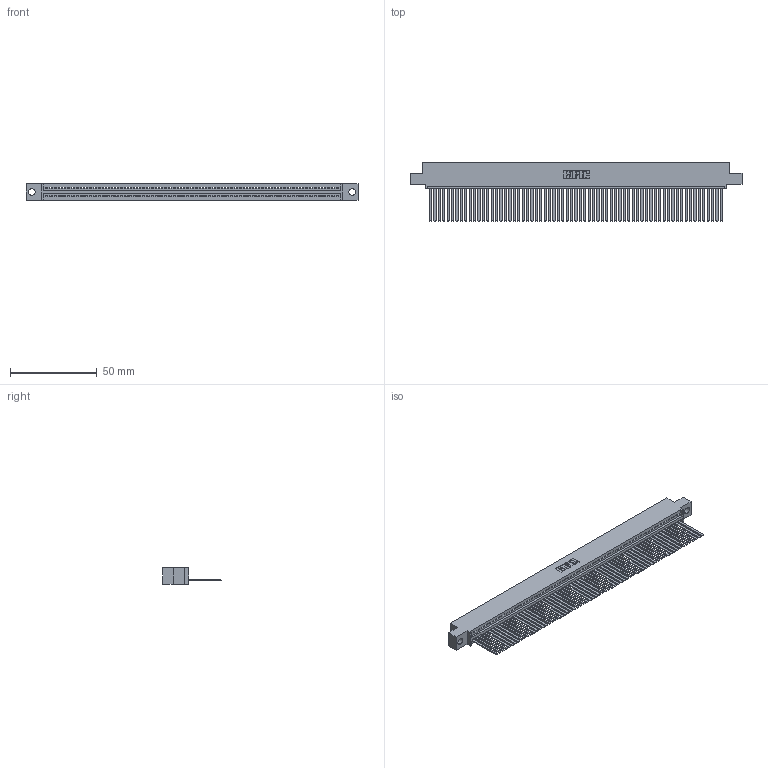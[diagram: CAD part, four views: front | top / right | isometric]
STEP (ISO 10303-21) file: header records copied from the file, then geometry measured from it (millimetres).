
FILE_DESCRIPTION (( 'STEP AP203' ), '1' );
FILE_NAME ('395-067-544-404.STEP', '2021-05-31T22:10:44', ( '' ), ( '' ), 'SwSTEP 2.0', 'SolidWorks 2020', '' );
FILE_SCHEMA (( 'CONFIG_CONTROL_DESIGN' ));
Length unit declared in the file: inch
Products named in the file (3): 345-292-001_345-293-144; 345 Part_0.110 Offset - 0.156 Dia-TI; 395-067-544-404
Assembly tree (68 placements, depth 2):
  395-067-544-404
    345 Part_0.110 Offset - 0.156 Dia-TI
    345-292-001_345-293-144  x67
Bounding box: 191.39 x 33.96 x 9.4 mm (x, y, z)
Volume: 18979.7 mm3; surface area: 27816 mm2
Topology: 68 solids, 68 shells, 3628 faces, 10975 edges, 7226 vertices
Faces by surface type: plane 2510, cylinder 1118
Entity records: 47427 total; most frequent: CARTESIAN_POINT 8223, ORIENTED_EDGE 8222, DIRECTION 7141, EDGE_CURVE 4111, LINE 3715, VECTOR 3715, VERTEX_POINT 2738, AXIS2_PLACEMENT_3D 1713
